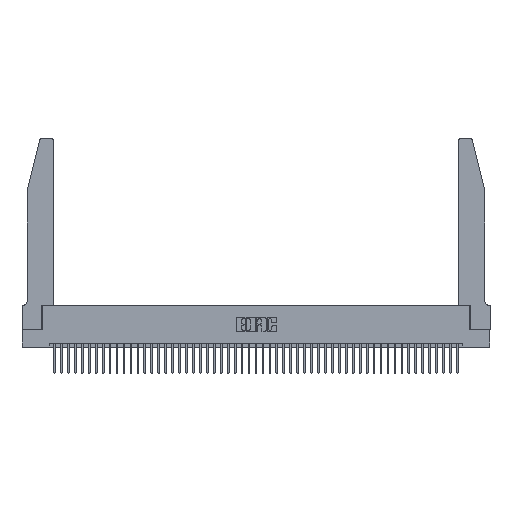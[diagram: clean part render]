
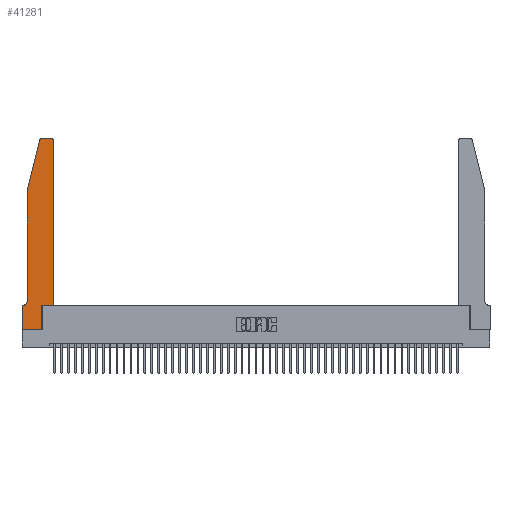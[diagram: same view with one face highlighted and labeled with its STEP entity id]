
A CAD part, top view. The second image highlights one B-rep face of the part: STEP entity #41281.
In plain terms, the highlighted planar face has unit normal (0, 0, 1).
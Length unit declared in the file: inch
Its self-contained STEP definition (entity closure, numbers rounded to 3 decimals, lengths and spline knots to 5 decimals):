
#458 = CARTESIAN_POINT ( 'NONE',  ( 0.0755, 2., 0.37 ) ) ;
#477 = ORIENTED_EDGE ( 'NONE', *, *, #22827, .T. ) ;
#888 = DIRECTION ( 'NONE',  ( -1., 0., 0. ) ) ;
#1445 = LINE ( 'NONE', #21994, #20337 ) ;
#2097 = EDGE_CURVE ( 'NONE', #17625, #11508, #12244, .T. ) ;
#2155 = VECTOR ( 'NONE', #37219, 39.37008 ) ;
#3644 = DIRECTION ( 'NONE',  ( 0., -1., 0. ) ) ;
#4466 = VERTEX_POINT ( 'NONE', #14161 ) ;
#4678 = CARTESIAN_POINT ( 'NONE',  ( 0.0755, 0.35, 0.37 ) ) ;
#4788 = CARTESIAN_POINT ( 'NONE',  ( 0.284, 2.75, 0.37 ) ) ;
#5050 = EDGE_CURVE ( 'NONE', #10058, #4466, #16726, .T. ) ;
#5469 = CARTESIAN_POINT ( 'NONE',  ( 0.4505, 2.72, 0.37 ) ) ;
#6184 = VERTEX_POINT ( 'NONE', #48215 ) ;
#6592 = AXIS2_PLACEMENT_3D ( 'NONE', #34941, #38875, #16364 ) ;
#6767 = VECTOR ( 'NONE', #3644, 39.37008 ) ;
#7349 = CARTESIAN_POINT ( 'NONE',  ( 0.0755, 2., 0.37 ) ) ;
#8073 = DIRECTION ( 'NONE',  ( 0., -1., 0. ) ) ;
#8449 = VECTOR ( 'NONE', #8073, 39.37008 ) ;
#9670 = LINE ( 'NONE', #458, #8449 ) ;
#10058 = VERTEX_POINT ( 'NONE', #4788 ) ;
#10668 = EDGE_CURVE ( 'NONE', #44170, #22709, #26081, .T. ) ;
#10810 = CARTESIAN_POINT ( 'NONE',  ( 0.284, 2.72, 0.37 ) ) ;
#11457 = VECTOR ( 'NONE', #35708, 39.37008 ) ;
#11508 = VERTEX_POINT ( 'NONE', #15701 ) ;
#12244 = LINE ( 'NONE', #40852, #2155 ) ;
#12373 = ORIENTED_EDGE ( 'NONE', *, *, #39750, .T. ) ;
#13305 = CARTESIAN_POINT ( 'NONE',  ( 0.2865, 0., 0.37 ) ) ;
#13540 = ORIENTED_EDGE ( 'NONE', *, *, #2097, .T. ) ;
#14117 = ORIENTED_EDGE ( 'NONE', *, *, #19956, .T. ) ;
#14161 = CARTESIAN_POINT ( 'NONE',  ( 0.25487, 2.72718, 0.37 ) ) ;
#14597 = DIRECTION ( 'NONE',  ( 1., 0., 0. ) ) ;
#15663 = LINE ( 'NONE', #24088, #16859 ) ;
#15701 = CARTESIAN_POINT ( 'NONE',  ( 0.4505, 0.35, 0.37 ) ) ;
#15900 = ORIENTED_EDGE ( 'NONE', *, *, #41637, .T. ) ;
#16057 = AXIS2_PLACEMENT_3D ( 'NONE', #10810, #37113, #14597 ) ;
#16364 = DIRECTION ( 'NONE',  ( 1., 0., 0. ) ) ;
#16668 = CARTESIAN_POINT ( 'NONE',  ( 0.2865, 0.35, 0.37 ) ) ;
#16726 = CIRCLE ( 'NONE', #16057, 0.03 ) ;
#16801 = LINE ( 'NONE', #29980, #6767 ) ;
#16859 = VECTOR ( 'NONE', #47262, 39.37008 ) ;
#17533 = CARTESIAN_POINT ( 'NONE',  ( 0.0755, 0.42, 0.37 ) ) ;
#17625 = VERTEX_POINT ( 'NONE', #16668 ) ;
#18092 = CARTESIAN_POINT ( 'NONE',  ( 0.0055, 0.42, 0.37 ) ) ;
#18448 = VERTEX_POINT ( 'NONE', #21383 ) ;
#18735 = DIRECTION ( 'NONE',  ( -0.239, -0.971, 0. ) ) ;
#19956 = EDGE_CURVE ( 'NONE', #18448, #35438, #9670, .T. ) ;
#20337 = VECTOR ( 'NONE', #25759, 39.37008 ) ;
#21383 = CARTESIAN_POINT ( 'NONE',  ( 0.0755, 2., 0.37 ) ) ;
#21889 = DIRECTION ( 'NONE',  ( -1., 0., 0. ) ) ;
#21994 = CARTESIAN_POINT ( 'NONE',  ( 0.2605, 2.75, 0.37 ) ) ;
#22050 = DIRECTION ( 'NONE',  ( 0., 0., 1. ) ) ;
#22696 = EDGE_CURVE ( 'NONE', #35438, #35784, #47070, .T. ) ;
#22709 = VERTEX_POINT ( 'NONE', #48182 ) ;
#22827 = EDGE_CURVE ( 'NONE', #4466, #18448, #32308, .T. ) ;
#24088 = CARTESIAN_POINT ( 'NONE',  ( 0., 0., 0.37 ) ) ;
#24519 = CARTESIAN_POINT ( 'NONE',  ( 0., 0., 0.37 ) ) ;
#25759 = DIRECTION ( 'NONE',  ( -1., 0., 0. ) ) ;
#26081 = CIRCLE ( 'NONE', #31966, 0.03 ) ;
#27531 = PLANE ( 'NONE',  #6592 ) ;
#29389 = ORIENTED_EDGE ( 'NONE', *, *, #5050, .T. ) ;
#29791 = EDGE_CURVE ( 'NONE', #36729, #17625, #41459, .T. ) ;
#29980 = CARTESIAN_POINT ( 'NONE',  ( 0., 0., 0.37 ) ) ;
#31328 = EDGE_LOOP ( 'NONE', ( #37048, #29389, #477, #14117, #44111, #47671, #38836, #12373, #42375, #13540, #15900, #35902 ) ) ;
#31709 = VECTOR ( 'NONE', #888, 39.37008 ) ;
#31966 = AXIS2_PLACEMENT_3D ( 'NONE', #44557, #22050, #48367 ) ;
#32308 = LINE ( 'NONE', #7349, #41158 ) ;
#32904 = LINE ( 'NONE', #4678, #31709 ) ;
#33123 = VECTOR ( 'NONE', #45076, 39.37008 ) ;
#34428 = CARTESIAN_POINT ( 'NONE',  ( 0.0055, 0.35, 0.37 ) ) ;
#34941 = CARTESIAN_POINT ( 'NONE',  ( 0., 0.35, 0.37 ) ) ;
#35438 = VERTEX_POINT ( 'NONE', #17533 ) ;
#35708 = DIRECTION ( 'NONE',  ( 0., 1., 0. ) ) ;
#35784 = VERTEX_POINT ( 'NONE', #34428 ) ;
#35902 = ORIENTED_EDGE ( 'NONE', *, *, #10668, .T. ) ;
#36729 = VERTEX_POINT ( 'NONE', #13305 ) ;
#37048 = ORIENTED_EDGE ( 'NONE', *, *, #39399, .T. ) ;
#37113 = DIRECTION ( 'NONE',  ( 0., 0., 1. ) ) ;
#37219 = DIRECTION ( 'NONE',  ( 1., 0., 0. ) ) ;
#37283 = FACE_OUTER_BOUND ( 'NONE', #31328, .T. ) ;
#38836 = ORIENTED_EDGE ( 'NONE', *, *, #39472, .T. ) ;
#38875 = DIRECTION ( 'NONE',  ( 0., 0., 1. ) ) ;
#39399 = EDGE_CURVE ( 'NONE', #22709, #10058, #1445, .T. ) ;
#39472 = EDGE_CURVE ( 'NONE', #6184, #47495, #16801, .T. ) ;
#39750 = EDGE_CURVE ( 'NONE', #47495, #36729, #15663, .T. ) ;
#40852 = CARTESIAN_POINT ( 'NONE',  ( 0.4505, 0.35, 0.37 ) ) ;
#41158 = VECTOR ( 'NONE', #18735, 39.37008 ) ;
#41281 = ADVANCED_FACE ( 'NONE', ( #37283 ), #27531, .T. ) ;
#41308 = CARTESIAN_POINT ( 'NONE',  ( 0.4505, 0.35, 0.37 ) ) ;
#41459 = LINE ( 'NONE', #43100, #11457 ) ;
#41637 = EDGE_CURVE ( 'NONE', #11508, #44170, #43123, .T. ) ;
#42375 = ORIENTED_EDGE ( 'NONE', *, *, #29791, .T. ) ;
#42983 = AXIS2_PLACEMENT_3D ( 'NONE', #18092, #44385, #21889 ) ;
#43100 = CARTESIAN_POINT ( 'NONE',  ( 0.2865, 0.35, 0.37 ) ) ;
#43123 = LINE ( 'NONE', #41308, #33123 ) ;
#44111 = ORIENTED_EDGE ( 'NONE', *, *, #22696, .T. ) ;
#44170 = VERTEX_POINT ( 'NONE', #5469 ) ;
#44385 = DIRECTION ( 'NONE',  ( 0., 0., -1. ) ) ;
#44557 = CARTESIAN_POINT ( 'NONE',  ( 0.4205, 2.72, 0.37 ) ) ;
#45076 = DIRECTION ( 'NONE',  ( 0., 1., 0. ) ) ;
#47070 = CIRCLE ( 'NONE', #42983, 0.07 ) ;
#47262 = DIRECTION ( 'NONE',  ( 1., 0., 0. ) ) ;
#47495 = VERTEX_POINT ( 'NONE', #24519 ) ;
#47671 = ORIENTED_EDGE ( 'NONE', *, *, #47982, .T. ) ;
#47982 = EDGE_CURVE ( 'NONE', #35784, #6184, #32904, .T. ) ;
#48182 = CARTESIAN_POINT ( 'NONE',  ( 0.4205, 2.75, 0.37 ) ) ;
#48215 = CARTESIAN_POINT ( 'NONE',  ( 0., 0.35, 0.37 ) ) ;
#48367 = DIRECTION ( 'NONE',  ( 1., 0., 0. ) ) ;
